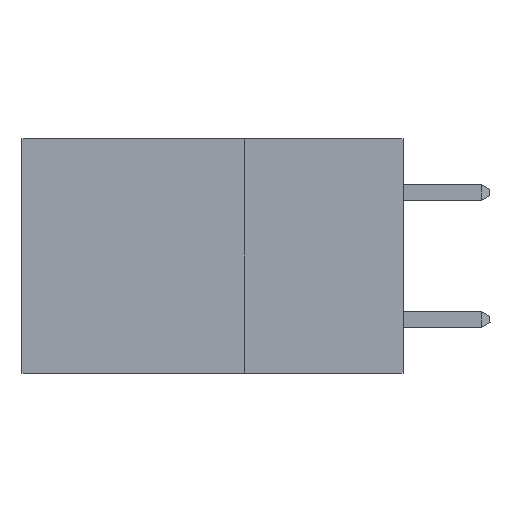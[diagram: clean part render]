
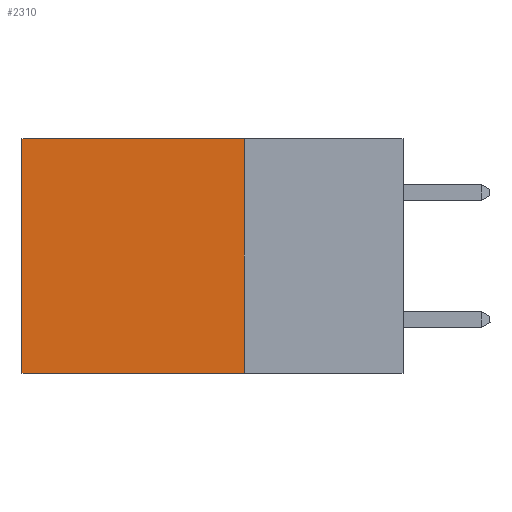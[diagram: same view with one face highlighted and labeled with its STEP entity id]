
A CAD part, left-side view. The second image highlights one B-rep face of the part: STEP entity #2310.
In plain terms, the highlighted planar face has unit normal (-1, 0, 0).
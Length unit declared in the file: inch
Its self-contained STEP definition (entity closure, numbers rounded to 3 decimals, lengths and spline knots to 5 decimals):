
#969 = EDGE_CURVE ( 'NONE', #1561, #6667, #9230, .T. ) ;
#1561 = VERTEX_POINT ( 'NONE', #9981 ) ;
#1624 = LINE ( 'NONE', #7766, #1984 ) ;
#1721 = CARTESIAN_POINT ( 'NONE',  ( 0.2875, 0.25, 0. ) ) ;
#1765 = DIRECTION ( 'NONE',  ( 0., 0., -1. ) ) ;
#1984 = VECTOR ( 'NONE', #3002, 39.37008 ) ;
#2310 = ADVANCED_FACE ( 'NONE', ( #9959 ), #7506, .F. ) ;
#2413 = LINE ( 'NONE', #5137, #10128 ) ;
#2675 = VECTOR ( 'NONE', #3852, 39.37008 ) ;
#2725 = DIRECTION ( 'NONE',  ( 0., 0., -1. ) ) ;
#2898 = ORIENTED_EDGE ( 'NONE', *, *, #3545, .F. ) ;
#3002 = DIRECTION ( 'NONE',  ( 0., 0., -1. ) ) ;
#3009 = CARTESIAN_POINT ( 'NONE',  ( 0.2875, 0.25, 0. ) ) ;
#3545 = EDGE_CURVE ( 'NONE', #7811, #9148, #1624, .T. ) ;
#3852 = DIRECTION ( 'NONE',  ( 0., 1., 0. ) ) ;
#3917 = ORIENTED_EDGE ( 'NONE', *, *, #969, .T. ) ;
#4051 = EDGE_LOOP ( 'NONE', ( #3917, #7407, #2898, #6795 ) ) ;
#4387 = DIRECTION ( 'NONE',  ( 1., 0., 0. ) ) ;
#4888 = CARTESIAN_POINT ( 'NONE',  ( 0.2875, 0.6, 0. ) ) ;
#5137 = CARTESIAN_POINT ( 'NONE',  ( 0.2875, 0.25, -0.37 ) ) ;
#5205 = DIRECTION ( 'NONE',  ( 0., 1., 0. ) ) ;
#5607 = CARTESIAN_POINT ( 'NONE',  ( 0.2875, 0.6, -0.37 ) ) ;
#5659 = AXIS2_PLACEMENT_3D ( 'NONE', #9740, #4387, #2725 ) ;
#5822 = VECTOR ( 'NONE', #1765, 39.37008 ) ;
#6667 = VERTEX_POINT ( 'NONE', #5607 ) ;
#6795 = ORIENTED_EDGE ( 'NONE', *, *, #7043, .T. ) ;
#7043 = EDGE_CURVE ( 'NONE', #7811, #1561, #8553, .T. ) ;
#7407 = ORIENTED_EDGE ( 'NONE', *, *, #8885, .F. ) ;
#7506 = PLANE ( 'NONE',  #5659 ) ;
#7766 = CARTESIAN_POINT ( 'NONE',  ( 0.2875, 0.25, 0. ) ) ;
#7811 = VERTEX_POINT ( 'NONE', #1721 ) ;
#8553 = LINE ( 'NONE', #3009, #2675 ) ;
#8885 = EDGE_CURVE ( 'NONE', #9148, #6667, #2413, .T. ) ;
#9148 = VERTEX_POINT ( 'NONE', #9444 ) ;
#9230 = LINE ( 'NONE', #4888, #5822 ) ;
#9444 = CARTESIAN_POINT ( 'NONE',  ( 0.2875, 0.25, -0.37 ) ) ;
#9740 = CARTESIAN_POINT ( 'NONE',  ( 0.2875, 0.25, 0. ) ) ;
#9959 = FACE_OUTER_BOUND ( 'NONE', #4051, .T. ) ;
#9981 = CARTESIAN_POINT ( 'NONE',  ( 0.2875, 0.6, 0. ) ) ;
#10128 = VECTOR ( 'NONE', #5205, 39.37008 ) ;
